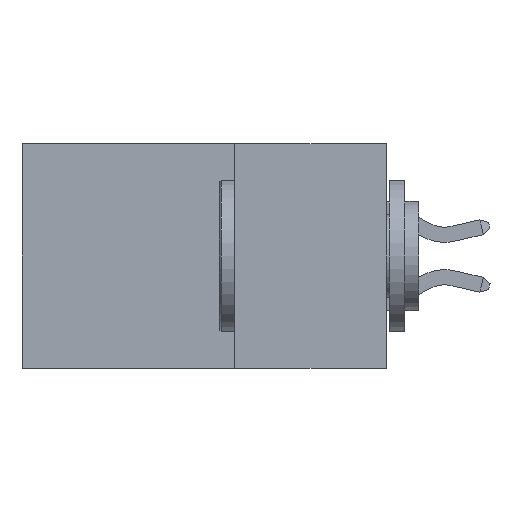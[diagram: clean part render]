
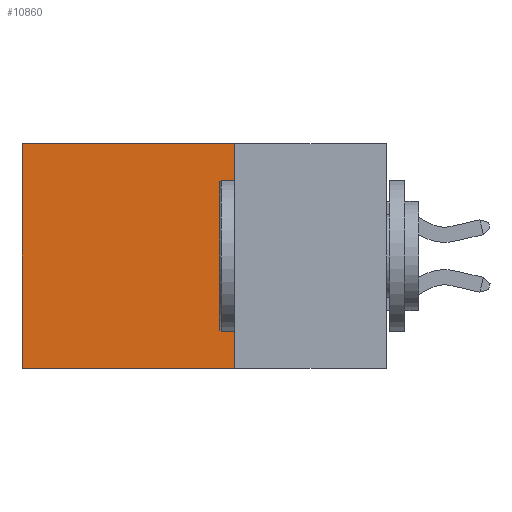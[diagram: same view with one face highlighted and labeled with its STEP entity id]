
A CAD part, left-side view. The second image highlights one B-rep face of the part: STEP entity #10860.
In plain terms, the highlighted planar face has unit normal (-1, 0, 0).
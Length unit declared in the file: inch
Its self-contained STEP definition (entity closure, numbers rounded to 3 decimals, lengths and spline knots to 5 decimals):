
#223 = VERTEX_POINT ( 'NONE', #5788 ) ;
#1193 = VECTOR ( 'NONE', #4707, 39.37008 ) ;
#1487 = VECTOR ( 'NONE', #8430, 39.37008 ) ;
#1673 = DIRECTION ( 'NONE',  ( 1., 0., 0. ) ) ;
#1934 = AXIS2_PLACEMENT_3D ( 'NONE', #9412, #1673, #4162 ) ;
#2098 = CARTESIAN_POINT ( 'NONE',  ( 0.298, 0.6, 0. ) ) ;
#2951 = ORIENTED_EDGE ( 'NONE', *, *, #10429, .F. ) ;
#3589 = VECTOR ( 'NONE', #14758, 39.37008 ) ;
#3962 = LINE ( 'NONE', #13261, #9628 ) ;
#4162 = DIRECTION ( 'NONE',  ( 0., 0., -1. ) ) ;
#4333 = ORIENTED_EDGE ( 'NONE', *, *, #11018, .T. ) ;
#4650 = EDGE_LOOP ( 'NONE', ( #10856, #2951, #7033, #4333 ) ) ;
#4707 = DIRECTION ( 'NONE',  ( 0., 1., 0. ) ) ;
#4739 = EDGE_CURVE ( 'NONE', #10699, #5870, #10386, .T. ) ;
#5770 = CARTESIAN_POINT ( 'NONE',  ( 0.298, 0.25, 0. ) ) ;
#5788 = CARTESIAN_POINT ( 'NONE',  ( 0.298, 0.25, 0. ) ) ;
#5870 = VERTEX_POINT ( 'NONE', #8680 ) ;
#6030 = CARTESIAN_POINT ( 'NONE',  ( 0.298, 0.25, -0.37 ) ) ;
#6874 = DIRECTION ( 'NONE',  ( 0., 0., -1. ) ) ;
#7033 = ORIENTED_EDGE ( 'NONE', *, *, #8556, .F. ) ;
#8430 = DIRECTION ( 'NONE',  ( 0., 0., -1. ) ) ;
#8556 = EDGE_CURVE ( 'NONE', #223, #14217, #3962, .T. ) ;
#8680 = CARTESIAN_POINT ( 'NONE',  ( 0.298, 0.6, -0.37 ) ) ;
#9412 = CARTESIAN_POINT ( 'NONE',  ( 0.298, 0.25, 0. ) ) ;
#9460 = LINE ( 'NONE', #5770, #3589 ) ;
#9628 = VECTOR ( 'NONE', #6874, 39.37008 ) ;
#10386 = LINE ( 'NONE', #2098, #1487 ) ;
#10429 = EDGE_CURVE ( 'NONE', #14217, #5870, #15310, .T. ) ;
#10699 = VERTEX_POINT ( 'NONE', #11649 ) ;
#10856 = ORIENTED_EDGE ( 'NONE', *, *, #4739, .T. ) ;
#10860 = ADVANCED_FACE ( 'NONE', ( #11478 ), #14405, .F. ) ;
#11018 = EDGE_CURVE ( 'NONE', #223, #10699, #9460, .T. ) ;
#11478 = FACE_OUTER_BOUND ( 'NONE', #4650, .T. ) ;
#11649 = CARTESIAN_POINT ( 'NONE',  ( 0.298, 0.6, 0. ) ) ;
#13261 = CARTESIAN_POINT ( 'NONE',  ( 0.298, 0.25, 0. ) ) ;
#14217 = VERTEX_POINT ( 'NONE', #16624 ) ;
#14405 = PLANE ( 'NONE',  #1934 ) ;
#14758 = DIRECTION ( 'NONE',  ( 0., 1., 0. ) ) ;
#15310 = LINE ( 'NONE', #6030, #1193 ) ;
#16624 = CARTESIAN_POINT ( 'NONE',  ( 0.298, 0.25, -0.37 ) ) ;
